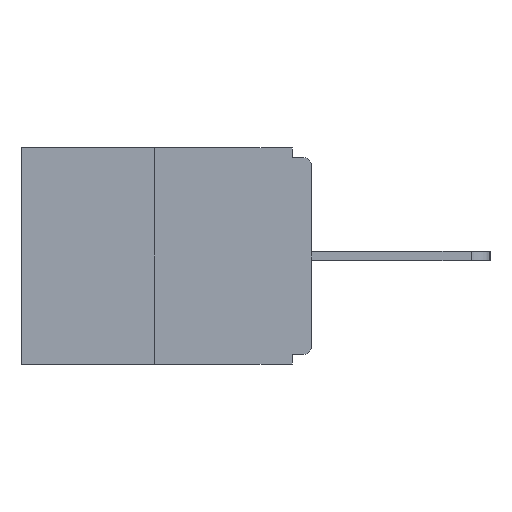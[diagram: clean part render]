
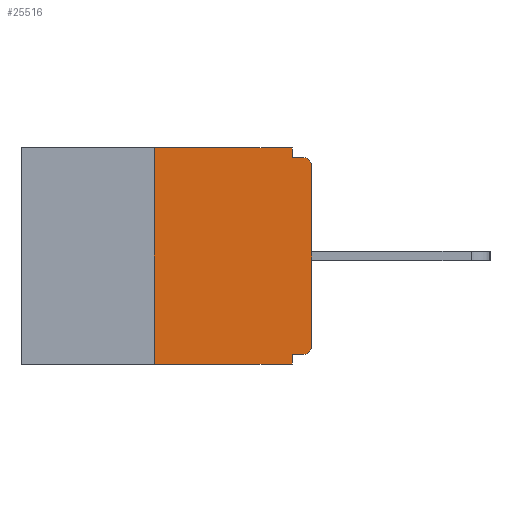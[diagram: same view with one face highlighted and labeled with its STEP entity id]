
A CAD part, left-side view. The second image highlights one B-rep face of the part: STEP entity #25516.
In plain terms, the highlighted planar face has unit normal (-1, 0, 0).
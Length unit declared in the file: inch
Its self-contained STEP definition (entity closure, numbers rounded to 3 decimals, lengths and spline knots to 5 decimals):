
#98 = ORIENTED_EDGE ( 'NONE', *, *, #18991, .T. ) ;
#416 = ORIENTED_EDGE ( 'NONE', *, *, #18651, .T. ) ;
#567 = DIRECTION ( 'NONE',  ( 0., 0., -1. ) ) ;
#1247 = DIRECTION ( 'NONE',  ( 0., -1., 0. ) ) ;
#1641 = CARTESIAN_POINT ( 'NONE',  ( 0., 0.031, -0.015 ) ) ;
#1719 = DIRECTION ( 'NONE',  ( 0., 0., -1. ) ) ;
#2308 = EDGE_CURVE ( 'NONE', #2748, #9359, #3512, .T. ) ;
#2748 = VERTEX_POINT ( 'NONE', #1641 ) ;
#3092 = VERTEX_POINT ( 'NONE', #23566 ) ;
#3143 = VERTEX_POINT ( 'NONE', #24559 ) ;
#3512 = LINE ( 'NONE', #19231, #24845 ) ;
#3850 = CIRCLE ( 'NONE', #9326, 0.015 ) ;
#4918 = LINE ( 'NONE', #5285, #25570 ) ;
#5285 = CARTESIAN_POINT ( 'NONE',  ( 0., 0., 0. ) ) ;
#6083 = DIRECTION ( 'NONE',  ( -1., 0., 0. ) ) ;
#6963 = DIRECTION ( 'NONE',  ( -1., 0., 0. ) ) ;
#7373 = VERTEX_POINT ( 'NONE', #10962 ) ;
#7546 = FACE_OUTER_BOUND ( 'NONE', #14335, .T. ) ;
#7655 = VECTOR ( 'NONE', #1247, 39.37008 ) ;
#7737 = ORIENTED_EDGE ( 'NONE', *, *, #17277, .F. ) ;
#8049 = CARTESIAN_POINT ( 'NONE',  ( 0., 0.015, -0.328 ) ) ;
#8142 = VECTOR ( 'NONE', #18938, 39.37008 ) ;
#8780 = LINE ( 'NONE', #8923, #8142 ) ;
#8923 = CARTESIAN_POINT ( 'NONE',  ( 0., 0., -0.328 ) ) ;
#9173 = VECTOR ( 'NONE', #21879, 39.37008 ) ;
#9292 = CARTESIAN_POINT ( 'NONE',  ( 0., 0.015, -0.015 ) ) ;
#9326 = AXIS2_PLACEMENT_3D ( 'NONE', #18049, #6083, #20100 ) ;
#9359 = VERTEX_POINT ( 'NONE', #9292 ) ;
#9882 = CARTESIAN_POINT ( 'NONE',  ( 0., 0.25, 0. ) ) ;
#10324 = VERTEX_POINT ( 'NONE', #9882 ) ;
#10412 = DIRECTION ( 'NONE',  ( 0., 0., 1. ) ) ;
#10962 = CARTESIAN_POINT ( 'NONE',  ( 0., 0., -0.313 ) ) ;
#12153 = ORIENTED_EDGE ( 'NONE', *, *, #15920, .F. ) ;
#12685 = CARTESIAN_POINT ( 'NONE',  ( 0., 0.031, -0.343 ) ) ;
#12943 = CIRCLE ( 'NONE', #22860, 0.015 ) ;
#12993 = LINE ( 'NONE', #25336, #7655 ) ;
#13106 = EDGE_CURVE ( 'NONE', #19361, #16813, #8780, .T. ) ;
#13144 = CARTESIAN_POINT ( 'NONE',  ( 0., 0.031, -0.328 ) ) ;
#13320 = DIRECTION ( 'NONE',  ( 0., 0., 1. ) ) ;
#13350 = ORIENTED_EDGE ( 'NONE', *, *, #18076, .F. ) ;
#13679 = ORIENTED_EDGE ( 'NONE', *, *, #13106, .F. ) ;
#13777 = DIRECTION ( 'NONE',  ( 1., 0., 0. ) ) ;
#13898 = VECTOR ( 'NONE', #567, 39.37008 ) ;
#14335 = EDGE_LOOP ( 'NONE', ( #13350, #25891, #416, #7737, #13679, #24379, #20327, #98, #16199, #12153 ) ) ;
#14517 = LINE ( 'NONE', #19856, #9173 ) ;
#15130 = DIRECTION ( 'NONE',  ( 0., -1., 0. ) ) ;
#15850 = VECTOR ( 'NONE', #22399, 39.37008 ) ;
#15920 = EDGE_CURVE ( 'NONE', #19701, #2748, #21228, .T. ) ;
#16199 = ORIENTED_EDGE ( 'NONE', *, *, #2308, .F. ) ;
#16388 = CARTESIAN_POINT ( 'NONE',  ( 0., 0.25, 0. ) ) ;
#16813 = VERTEX_POINT ( 'NONE', #13144 ) ;
#17277 = EDGE_CURVE ( 'NONE', #16813, #3092, #19265, .T. ) ;
#18049 = CARTESIAN_POINT ( 'NONE',  ( 0., 0.015, -0.313 ) ) ;
#18076 = EDGE_CURVE ( 'NONE', #10324, #19701, #12993, .T. ) ;
#18651 = EDGE_CURVE ( 'NONE', #25701, #3092, #14517, .T. ) ;
#18938 = DIRECTION ( 'NONE',  ( 0., 1., 0. ) ) ;
#18957 = CARTESIAN_POINT ( 'NONE',  ( 0., 0.015, -0.03 ) ) ;
#18991 = EDGE_CURVE ( 'NONE', #3143, #9359, #12943, .T. ) ;
#19231 = CARTESIAN_POINT ( 'NONE',  ( 0., 0., -0.015 ) ) ;
#19265 = LINE ( 'NONE', #12685, #13898 ) ;
#19361 = VERTEX_POINT ( 'NONE', #8049 ) ;
#19701 = VERTEX_POINT ( 'NONE', #21203 ) ;
#19760 = PLANE ( 'NONE',  #20818 ) ;
#19856 = CARTESIAN_POINT ( 'NONE',  ( 0., 0.46, -0.343 ) ) ;
#20100 = DIRECTION ( 'NONE',  ( 0., 0., -1. ) ) ;
#20327 = ORIENTED_EDGE ( 'NONE', *, *, #22529, .T. ) ;
#20385 = CARTESIAN_POINT ( 'NONE',  ( 0., 0.25, -0.343 ) ) ;
#20818 = AXIS2_PLACEMENT_3D ( 'NONE', #25766, #13777, #1719 ) ;
#20977 = DIRECTION ( 'NONE',  ( 0., 0., -1. ) ) ;
#21203 = CARTESIAN_POINT ( 'NONE',  ( 0., 0.031, 0. ) ) ;
#21228 = LINE ( 'NONE', #22311, #15850 ) ;
#21879 = DIRECTION ( 'NONE',  ( 0., -1., 0. ) ) ;
#22077 = VECTOR ( 'NONE', #10412, 39.37008 ) ;
#22311 = CARTESIAN_POINT ( 'NONE',  ( 0., 0.031, 0. ) ) ;
#22399 = DIRECTION ( 'NONE',  ( 0., 0., -1. ) ) ;
#22529 = EDGE_CURVE ( 'NONE', #7373, #3143, #4918, .T. ) ;
#22687 = LINE ( 'NONE', #16388, #22077 ) ;
#22860 = AXIS2_PLACEMENT_3D ( 'NONE', #18957, #6963, #20977 ) ;
#23566 = CARTESIAN_POINT ( 'NONE',  ( 0., 0.031, -0.343 ) ) ;
#24007 = EDGE_CURVE ( 'NONE', #25701, #10324, #22687, .T. ) ;
#24371 = EDGE_CURVE ( 'NONE', #19361, #7373, #3850, .T. ) ;
#24379 = ORIENTED_EDGE ( 'NONE', *, *, #24371, .T. ) ;
#24559 = CARTESIAN_POINT ( 'NONE',  ( 0., 0., -0.03 ) ) ;
#24845 = VECTOR ( 'NONE', #15130, 39.37008 ) ;
#25336 = CARTESIAN_POINT ( 'NONE',  ( 0., 0.46, 0. ) ) ;
#25516 = ADVANCED_FACE ( 'NONE', ( #7546 ), #19760, .F. ) ;
#25570 = VECTOR ( 'NONE', #13320, 39.37008 ) ;
#25701 = VERTEX_POINT ( 'NONE', #20385 ) ;
#25766 = CARTESIAN_POINT ( 'NONE',  ( 0., 0.46, 0. ) ) ;
#25891 = ORIENTED_EDGE ( 'NONE', *, *, #24007, .F. ) ;
